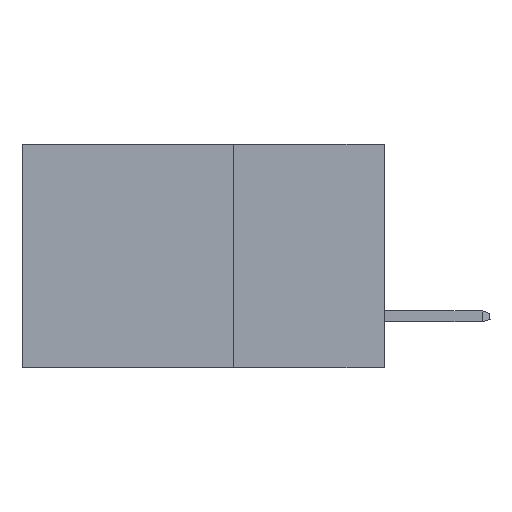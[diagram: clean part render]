
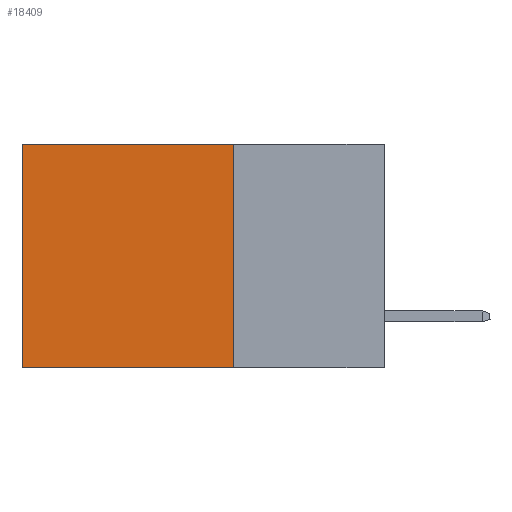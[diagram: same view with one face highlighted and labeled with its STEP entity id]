
A CAD part, left-side view. The second image highlights one B-rep face of the part: STEP entity #18409.
In plain terms, the highlighted planar face has unit normal (-1, 0, 0).
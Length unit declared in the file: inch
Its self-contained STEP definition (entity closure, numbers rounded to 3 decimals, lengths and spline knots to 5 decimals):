
#654 = LINE ( 'NONE', #11862, #2724 ) ;
#724 = LINE ( 'NONE', #7173, #1892 ) ;
#746 = DIRECTION ( 'NONE',  ( 0., 0., -1. ) ) ;
#1892 = VECTOR ( 'NONE', #2462, 39.37008 ) ;
#2182 = CARTESIAN_POINT ( 'NONE',  ( 0.298, 0.25, 0. ) ) ;
#2262 = PLANE ( 'NONE',  #6153 ) ;
#2462 = DIRECTION ( 'NONE',  ( 0., 0., -1. ) ) ;
#2511 = LINE ( 'NONE', #13285, #11749 ) ;
#2724 = VECTOR ( 'NONE', #2823, 39.37008 ) ;
#2823 = DIRECTION ( 'NONE',  ( 0., 1., 0. ) ) ;
#2895 = EDGE_LOOP ( 'NONE', ( #10331, #17000, #18458, #9328 ) ) ;
#3213 = EDGE_CURVE ( 'NONE', #16986, #12015, #2511, .T. ) ;
#4839 = EDGE_CURVE ( 'NONE', #18343, #17675, #654, .T. ) ;
#5383 = FACE_OUTER_BOUND ( 'NONE', #2895, .T. ) ;
#6153 = AXIS2_PLACEMENT_3D ( 'NONE', #18299, #12577, #9545 ) ;
#7173 = CARTESIAN_POINT ( 'NONE',  ( 0.298, 0.6, 0. ) ) ;
#7880 = CARTESIAN_POINT ( 'NONE',  ( 0.298, 0.6, 0. ) ) ;
#8058 = CARTESIAN_POINT ( 'NONE',  ( 0.298, 0.25, -0.37 ) ) ;
#8479 = EDGE_CURVE ( 'NONE', #16986, #18343, #13242, .T. ) ;
#9328 = ORIENTED_EDGE ( 'NONE', *, *, #3213, .T. ) ;
#9545 = DIRECTION ( 'NONE',  ( 0., 0., -1. ) ) ;
#10331 = ORIENTED_EDGE ( 'NONE', *, *, #15496, .T. ) ;
#11749 = VECTOR ( 'NONE', #16010, 39.37008 ) ;
#11862 = CARTESIAN_POINT ( 'NONE',  ( 0.298, 0.25, -0.37 ) ) ;
#12015 = VERTEX_POINT ( 'NONE', #7880 ) ;
#12577 = DIRECTION ( 'NONE',  ( 1., 0., 0. ) ) ;
#12597 = CARTESIAN_POINT ( 'NONE',  ( 0.298, 0.6, -0.37 ) ) ;
#13242 = LINE ( 'NONE', #2182, #17577 ) ;
#13285 = CARTESIAN_POINT ( 'NONE',  ( 0.298, 0.25, 0. ) ) ;
#14086 = CARTESIAN_POINT ( 'NONE',  ( 0.298, 0.25, 0. ) ) ;
#15496 = EDGE_CURVE ( 'NONE', #12015, #17675, #724, .T. ) ;
#16010 = DIRECTION ( 'NONE',  ( 0., 1., 0. ) ) ;
#16986 = VERTEX_POINT ( 'NONE', #14086 ) ;
#17000 = ORIENTED_EDGE ( 'NONE', *, *, #4839, .F. ) ;
#17577 = VECTOR ( 'NONE', #746, 39.37008 ) ;
#17675 = VERTEX_POINT ( 'NONE', #12597 ) ;
#18299 = CARTESIAN_POINT ( 'NONE',  ( 0.298, 0.25, 0. ) ) ;
#18343 = VERTEX_POINT ( 'NONE', #8058 ) ;
#18409 = ADVANCED_FACE ( 'NONE', ( #5383 ), #2262, .F. ) ;
#18458 = ORIENTED_EDGE ( 'NONE', *, *, #8479, .F. ) ;
